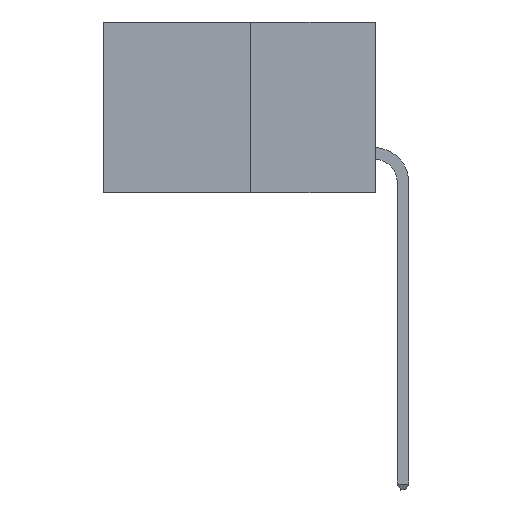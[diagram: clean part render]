
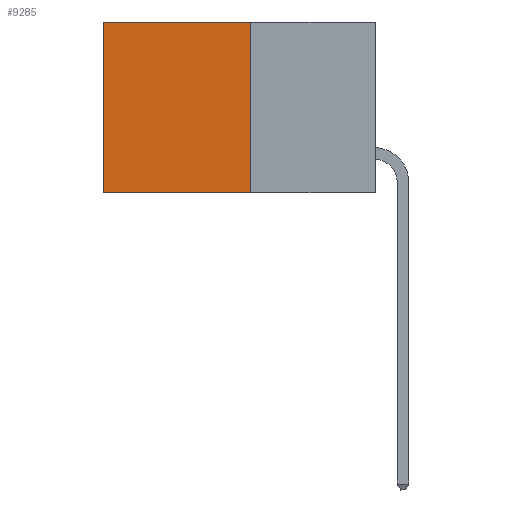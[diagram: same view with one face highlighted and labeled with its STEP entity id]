
A CAD part, left-side view. The second image highlights one B-rep face of the part: STEP entity #9285.
In plain terms, the highlighted planar face has unit normal (-1, 0, 0).
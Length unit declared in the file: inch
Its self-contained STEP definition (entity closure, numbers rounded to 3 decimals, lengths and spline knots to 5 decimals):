
#1061 = LINE ( 'NONE', #15141, #16217 ) ;
#2750 = ORIENTED_EDGE ( 'NONE', *, *, #18102, .F. ) ;
#2810 = CARTESIAN_POINT ( 'NONE',  ( 0.277, 0.59, -0.37 ) ) ;
#3292 = LINE ( 'NONE', #2810, #7992 ) ;
#3395 = VECTOR ( 'NONE', #15407, 39.37008 ) ;
#3551 = EDGE_CURVE ( 'NONE', #4958, #9292, #3292, .T. ) ;
#4840 = EDGE_CURVE ( 'NONE', #12052, #4958, #8883, .T. ) ;
#4958 = VERTEX_POINT ( 'NONE', #23865 ) ;
#6363 = FACE_OUTER_BOUND ( 'NONE', #14408, .T. ) ;
#7626 = CARTESIAN_POINT ( 'NONE',  ( 0.277, 0.27, -0.37 ) ) ;
#7944 = ORIENTED_EDGE ( 'NONE', *, *, #3551, .T. ) ;
#7992 = VECTOR ( 'NONE', #21072, 39.37008 ) ;
#8883 = LINE ( 'NONE', #25183, #19241 ) ;
#9285 = ADVANCED_FACE ( 'NONE', ( #6363 ), #14033, .F. ) ;
#9292 = VERTEX_POINT ( 'NONE', #13829 ) ;
#10063 = AXIS2_PLACEMENT_3D ( 'NONE', #13987, #13921, #13879 ) ;
#11283 = ORIENTED_EDGE ( 'NONE', *, *, #20980, .F. ) ;
#12052 = VERTEX_POINT ( 'NONE', #12271 ) ;
#12271 = CARTESIAN_POINT ( 'NONE',  ( 0.277, 0.27, 0. ) ) ;
#13829 = CARTESIAN_POINT ( 'NONE',  ( 0.277, 0.59, -0.37 ) ) ;
#13879 = DIRECTION ( 'NONE',  ( 0., 0., -1. ) ) ;
#13921 = DIRECTION ( 'NONE',  ( 1., 0., 0. ) ) ;
#13987 = CARTESIAN_POINT ( 'NONE',  ( 0.277, 0.27, -0.37 ) ) ;
#14033 = PLANE ( 'NONE',  #10063 ) ;
#14408 = EDGE_LOOP ( 'NONE', ( #7944, #2750, #11283, #15080 ) ) ;
#15080 = ORIENTED_EDGE ( 'NONE', *, *, #4840, .T. ) ;
#15141 = CARTESIAN_POINT ( 'NONE',  ( 0.277, 0.27, -0.37 ) ) ;
#15407 = DIRECTION ( 'NONE',  ( 0., 0., -1. ) ) ;
#16217 = VECTOR ( 'NONE', #17123, 39.37008 ) ;
#17123 = DIRECTION ( 'NONE',  ( 0., 1., 0. ) ) ;
#18102 = EDGE_CURVE ( 'NONE', #24000, #9292, #1061, .T. ) ;
#18466 = LINE ( 'NONE', #7626, #3395 ) ;
#19241 = VECTOR ( 'NONE', #25176, 39.37008 ) ;
#19262 = CARTESIAN_POINT ( 'NONE',  ( 0.277, 0.27, -0.37 ) ) ;
#20980 = EDGE_CURVE ( 'NONE', #12052, #24000, #18466, .T. ) ;
#21072 = DIRECTION ( 'NONE',  ( 0., 0., -1. ) ) ;
#23865 = CARTESIAN_POINT ( 'NONE',  ( 0.277, 0.59, 0. ) ) ;
#24000 = VERTEX_POINT ( 'NONE', #19262 ) ;
#25176 = DIRECTION ( 'NONE',  ( 0., 1., 0. ) ) ;
#25183 = CARTESIAN_POINT ( 'NONE',  ( 0.277, 0.27, 0. ) ) ;
